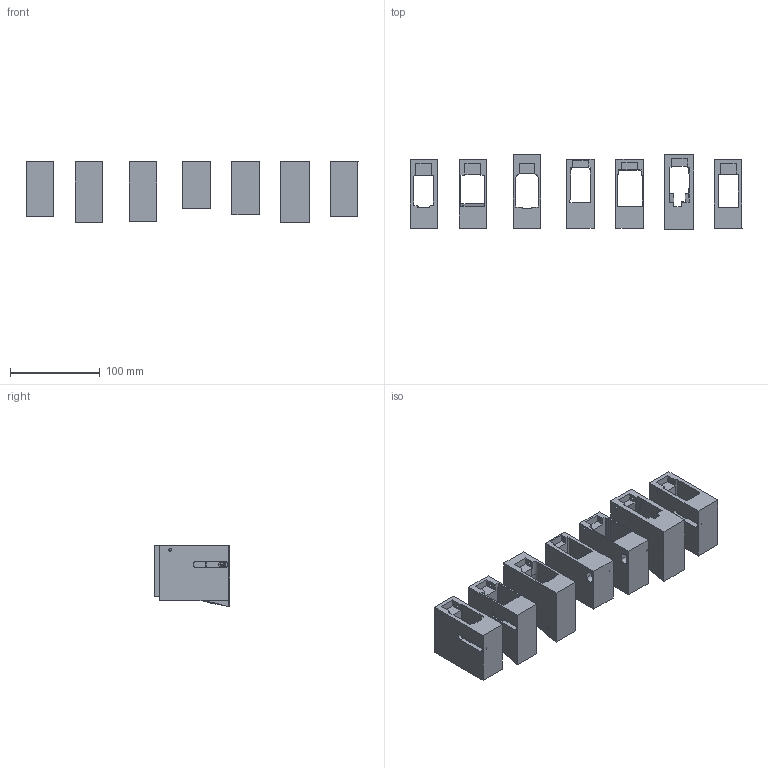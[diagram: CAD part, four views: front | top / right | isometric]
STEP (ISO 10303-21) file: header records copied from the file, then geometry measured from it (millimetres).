
FILE_DESCRIPTION(/* description */ (''),/* implementation_level */ '2;1');
FILE_NAME(/* name */ 'PCC 1.0/STEP/Magwells/Magwell Pack #1.step',/* time_stamp */ '2022-04-06T16:05:49-04:00',/* author */ (''),/* organization */ (''),/* preprocessor_version */ 'ST-DEVELOPER v18.1',/* originating_system */ 'Autodesk Translation Framework v10.14.0.1471',/* authorisation */ '');
FILE_SCHEMA (('AUTOMOTIVE_DESIGN { 1 0 10303 214 3 1 1 }'));
Length unit declared in the file: millimetre
Products named in the file (18): #11497; 7.62x25 (1); PPS43 Magwell; Frame (7); 45 ACP (1); Macon Armory Magwell; Magwell; M3 Grease Gun Magwell; Frame (4) (1) (1) (1); 9MM (1); AR-9 Colt Magwell; Frame (5) (4); Sten Magwell; Frame (1) (1); MP5 Magwell; Frame (6) (1) (1); Vityas Magwell; Frame (6) (2)
Assembly tree (17 placements, depth 4):
  #11497
    7.62x25 (1)
      PPS43 Magwell
        Frame (7)
    45 ACP (1)
      Macon Armory Magwell
        Magwell
      M3 Grease Gun Magwell
        Frame (4) (1) (1) (1)
    9MM (1)
      AR-9 Colt Magwell
        Frame (5) (4)
      Sten Magwell
        Frame (1) (1)
      MP5 Magwell
        Frame (6) (1) (1)
      Vityas Magwell
        Frame (6) (2)
Bounding box: 370.68 x 83.95 x 68.29 mm (x, y, z)
Volume: 583035.7 mm3; surface area: 171893.5 mm2
Topology: 7 solids, 7 shells, 315 faces, 885 edges, 592 vertices
Faces by surface type: plane 189, cylinder 93, bspline 31, torus 2
Full cylindrical faces by diameter (mm): 3 x17, 4.5 x1, 5.182 x5, 7 x1, 7.938 x5
Entity records: 11527 total; most frequent: CARTESIAN_POINT 2731, ORIENTED_EDGE 1770, DIRECTION 1734, EDGE_CURVE 885, LINE 614, VECTOR 614, VERTEX_POINT 592, AXIS2_PLACEMENT_3D 560
